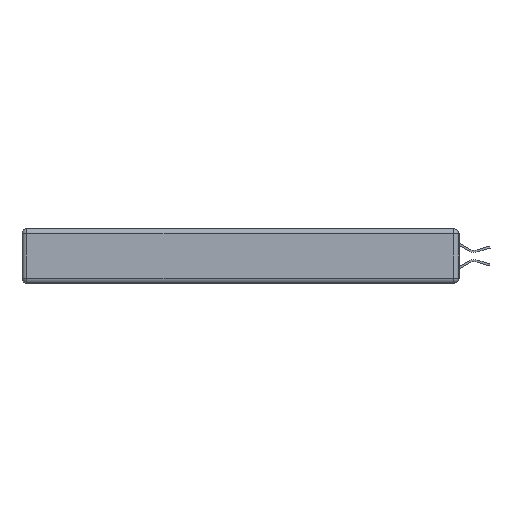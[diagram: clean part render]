
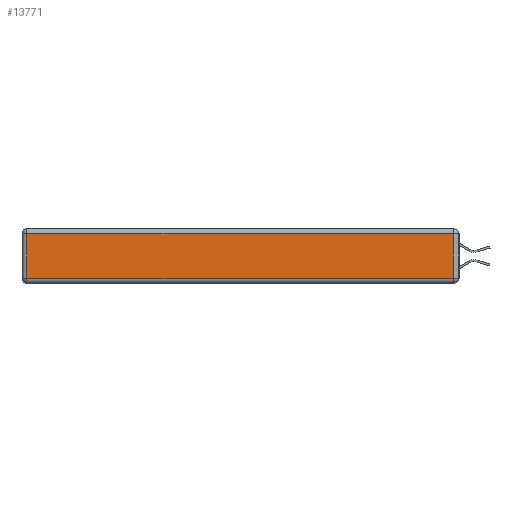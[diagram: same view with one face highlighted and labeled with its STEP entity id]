
A CAD part, left-side view. The second image highlights one B-rep face of the part: STEP entity #13771.
In plain terms, the highlighted planar face has unit normal (-1, 0, 0).
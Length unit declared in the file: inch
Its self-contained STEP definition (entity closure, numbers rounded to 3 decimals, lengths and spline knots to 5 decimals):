
#697 = EDGE_CURVE ( 'NONE', #6325, #4760, #9645, .T. ) ;
#965 = CARTESIAN_POINT ( 'NONE',  ( 0., 0., -0.313 ) ) ;
#1481 = DIRECTION ( 'NONE',  ( 0., 0., 1. ) ) ;
#2078 = EDGE_LOOP ( 'NONE', ( #12462, #10863, #6560, #9286 ) ) ;
#2161 = DIRECTION ( 'NONE',  ( 0., 1., 0. ) ) ;
#2287 = CARTESIAN_POINT ( 'NONE',  ( 0., 0.03, -0.03 ) ) ;
#2298 = CARTESIAN_POINT ( 'NONE',  ( 0., 2.75, -0.03 ) ) ;
#2374 = VECTOR ( 'NONE', #14100, 39.37008 ) ;
#2572 = DIRECTION ( 'NONE',  ( 0., 0., 1. ) ) ;
#2994 = VECTOR ( 'NONE', #12561, 39.37008 ) ;
#3203 = CARTESIAN_POINT ( 'NONE',  ( 0., 0.03, -0.313 ) ) ;
#3886 = LINE ( 'NONE', #6283, #2994 ) ;
#4080 = EDGE_CURVE ( 'NONE', #8683, #6325, #3886, .T. ) ;
#4488 = EDGE_CURVE ( 'NONE', #4760, #13787, #7895, .T. ) ;
#4760 = VERTEX_POINT ( 'NONE', #3203 ) ;
#5882 = DIRECTION ( 'NONE',  ( -1., 0., 0. ) ) ;
#6283 = CARTESIAN_POINT ( 'NONE',  ( 0., 2.72, -0.343 ) ) ;
#6325 = VERTEX_POINT ( 'NONE', #9430 ) ;
#6560 = ORIENTED_EDGE ( 'NONE', *, *, #8247, .T. ) ;
#6947 = CARTESIAN_POINT ( 'NONE',  ( 0., 0.03, -0.343 ) ) ;
#7567 = VECTOR ( 'NONE', #2161, 39.37008 ) ;
#7895 = LINE ( 'NONE', #6947, #10395 ) ;
#8115 = PLANE ( 'NONE',  #12208 ) ;
#8247 = EDGE_CURVE ( 'NONE', #13787, #8683, #11932, .T. ) ;
#8683 = VERTEX_POINT ( 'NONE', #9301 ) ;
#9286 = ORIENTED_EDGE ( 'NONE', *, *, #4080, .T. ) ;
#9301 = CARTESIAN_POINT ( 'NONE',  ( 0., 2.72, -0.03 ) ) ;
#9430 = CARTESIAN_POINT ( 'NONE',  ( 0., 2.72, -0.313 ) ) ;
#9645 = LINE ( 'NONE', #965, #2374 ) ;
#10395 = VECTOR ( 'NONE', #1481, 39.37008 ) ;
#10863 = ORIENTED_EDGE ( 'NONE', *, *, #4488, .T. ) ;
#11046 = CARTESIAN_POINT ( 'NONE',  ( 0., 0., -0.343 ) ) ;
#11932 = LINE ( 'NONE', #2298, #7567 ) ;
#12208 = AXIS2_PLACEMENT_3D ( 'NONE', #11046, #5882, #2572 ) ;
#12260 = FACE_OUTER_BOUND ( 'NONE', #2078, .T. ) ;
#12462 = ORIENTED_EDGE ( 'NONE', *, *, #697, .T. ) ;
#12561 = DIRECTION ( 'NONE',  ( 0., 0., -1. ) ) ;
#13771 = ADVANCED_FACE ( 'NONE', ( #12260 ), #8115, .T. ) ;
#13787 = VERTEX_POINT ( 'NONE', #2287 ) ;
#14100 = DIRECTION ( 'NONE',  ( 0., -1., 0. ) ) ;
